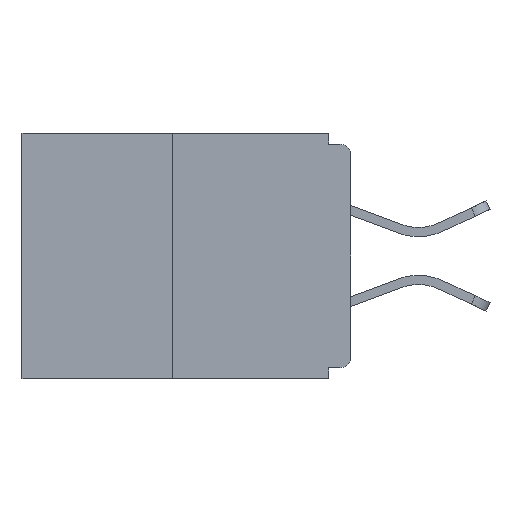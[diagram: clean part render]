
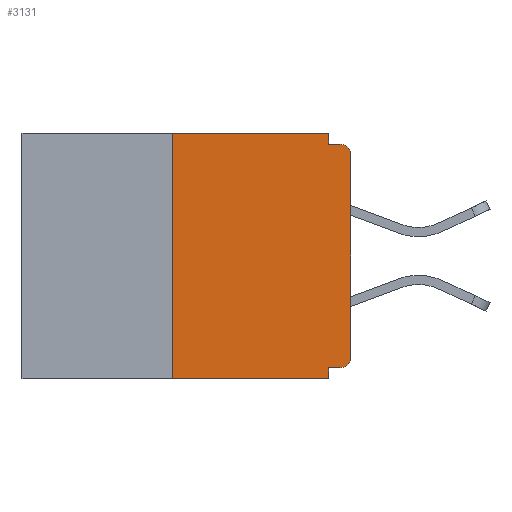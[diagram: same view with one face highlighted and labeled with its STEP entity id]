
A CAD part, left-side view. The second image highlights one B-rep face of the part: STEP entity #3131.
In plain terms, the highlighted planar face has unit normal (-1, 0, 0).
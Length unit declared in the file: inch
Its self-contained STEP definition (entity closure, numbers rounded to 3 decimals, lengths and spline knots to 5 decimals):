
#5 = DIRECTION ( 'NONE',  ( 0., 0., -1. ) ) ;
#140 = CARTESIAN_POINT ( 'NONE',  ( 0., 0.015, -0.03 ) ) ;
#191 = DIRECTION ( 'NONE',  ( 0., 0., -1. ) ) ;
#208 = CARTESIAN_POINT ( 'NONE',  ( 0., 0., -0.313 ) ) ;
#235 = VECTOR ( 'NONE', #4540, 39.37008 ) ;
#478 = EDGE_CURVE ( 'NONE', #4354, #5732, #7126, .T. ) ;
#539 = DIRECTION ( 'NONE',  ( 0., -1., 0. ) ) ;
#550 = EDGE_CURVE ( 'NONE', #5546, #5418, #6744, .T. ) ;
#612 = LINE ( 'NONE', #3067, #3023 ) ;
#686 = ORIENTED_EDGE ( 'NONE', *, *, #10364, .T. ) ;
#1331 = CARTESIAN_POINT ( 'NONE',  ( 0., 0.25, 0. ) ) ;
#1638 = VECTOR ( 'NONE', #6663, 39.37008 ) ;
#1967 = VERTEX_POINT ( 'NONE', #8378 ) ;
#2022 = CIRCLE ( 'NONE', #10120, 0.015 ) ;
#2124 = LINE ( 'NONE', #14376, #12943 ) ;
#2275 = ORIENTED_EDGE ( 'NONE', *, *, #2894, .T. ) ;
#2577 = DIRECTION ( 'NONE',  ( 1., 0., 0. ) ) ;
#2894 = EDGE_CURVE ( 'NONE', #5546, #4735, #2022, .T. ) ;
#2898 = CARTESIAN_POINT ( 'NONE',  ( 0., 0.015, -0.015 ) ) ;
#3023 = VECTOR ( 'NONE', #10588, 39.37008 ) ;
#3067 = CARTESIAN_POINT ( 'NONE',  ( 0., 0.25, 0. ) ) ;
#3131 = ADVANCED_FACE ( 'NONE', ( #10242 ), #11350, .F. ) ;
#3276 = VERTEX_POINT ( 'NONE', #9577 ) ;
#3657 = CARTESIAN_POINT ( 'NONE',  ( 0., 0., -0.015 ) ) ;
#3963 = DIRECTION ( 'NONE',  ( -1., 0., 0. ) ) ;
#4160 = VERTEX_POINT ( 'NONE', #7497 ) ;
#4187 = CARTESIAN_POINT ( 'NONE',  ( 0., 0.015, -0.313 ) ) ;
#4350 = VECTOR ( 'NONE', #9891, 39.37008 ) ;
#4354 = VERTEX_POINT ( 'NONE', #1331 ) ;
#4540 = DIRECTION ( 'NONE',  ( 0., 0., 1. ) ) ;
#4735 = VERTEX_POINT ( 'NONE', #208 ) ;
#5418 = VERTEX_POINT ( 'NONE', #10312 ) ;
#5546 = VERTEX_POINT ( 'NONE', #13089 ) ;
#5732 = VERTEX_POINT ( 'NONE', #11328 ) ;
#5743 = DIRECTION ( 'NONE',  ( 0., 0., -1. ) ) ;
#5886 = CARTESIAN_POINT ( 'NONE',  ( 0., 0.031, 0. ) ) ;
#5913 = ORIENTED_EDGE ( 'NONE', *, *, #6759, .F. ) ;
#5935 = ORIENTED_EDGE ( 'NONE', *, *, #11671, .T. ) ;
#6023 = ORIENTED_EDGE ( 'NONE', *, *, #550, .F. ) ;
#6123 = VECTOR ( 'NONE', #539, 39.37008 ) ;
#6312 = CARTESIAN_POINT ( 'NONE',  ( 0., 0.46, 0. ) ) ;
#6349 = ORIENTED_EDGE ( 'NONE', *, *, #6491, .F. ) ;
#6491 = EDGE_CURVE ( 'NONE', #5418, #1967, #7750, .T. ) ;
#6597 = CARTESIAN_POINT ( 'NONE',  ( 0., 0., -0.328 ) ) ;
#6663 = DIRECTION ( 'NONE',  ( 0., 0., -1. ) ) ;
#6671 = VECTOR ( 'NONE', #5743, 39.37008 ) ;
#6744 = LINE ( 'NONE', #6597, #4350 ) ;
#6759 = EDGE_CURVE ( 'NONE', #7288, #4354, #612, .T. ) ;
#6801 = EDGE_LOOP ( 'NONE', ( #8168, #5913, #686, #6349, #6023, #2275, #5935, #8076, #10536, #8285 ) ) ;
#7126 = LINE ( 'NONE', #6312, #10407 ) ;
#7288 = VERTEX_POINT ( 'NONE', #9785 ) ;
#7497 = CARTESIAN_POINT ( 'NONE',  ( 0., 0., -0.03 ) ) ;
#7750 = LINE ( 'NONE', #7894, #1638 ) ;
#7894 = CARTESIAN_POINT ( 'NONE',  ( 0., 0.031, -0.343 ) ) ;
#8076 = ORIENTED_EDGE ( 'NONE', *, *, #10401, .T. ) ;
#8155 = DIRECTION ( 'NONE',  ( 0., -1., 0. ) ) ;
#8168 = ORIENTED_EDGE ( 'NONE', *, *, #478, .F. ) ;
#8184 = EDGE_CURVE ( 'NONE', #3276, #13270, #10516, .T. ) ;
#8285 = ORIENTED_EDGE ( 'NONE', *, *, #14337, .F. ) ;
#8350 = LINE ( 'NONE', #5886, #6671 ) ;
#8378 = CARTESIAN_POINT ( 'NONE',  ( 0., 0.031, -0.343 ) ) ;
#8497 = AXIS2_PLACEMENT_3D ( 'NONE', #140, #13277, #5 ) ;
#8645 = DIRECTION ( 'NONE',  ( 0., 0., -1. ) ) ;
#9577 = CARTESIAN_POINT ( 'NONE',  ( 0., 0.031, -0.015 ) ) ;
#9785 = CARTESIAN_POINT ( 'NONE',  ( 0., 0.25, -0.343 ) ) ;
#9891 = DIRECTION ( 'NONE',  ( 0., 1., 0. ) ) ;
#10120 = AXIS2_PLACEMENT_3D ( 'NONE', #4187, #3963, #8645 ) ;
#10141 = CIRCLE ( 'NONE', #8497, 0.015 ) ;
#10242 = FACE_OUTER_BOUND ( 'NONE', #6801, .T. ) ;
#10312 = CARTESIAN_POINT ( 'NONE',  ( 0., 0.031, -0.328 ) ) ;
#10319 = CARTESIAN_POINT ( 'NONE',  ( 0., 0., 0. ) ) ;
#10364 = EDGE_CURVE ( 'NONE', #7288, #1967, #2124, .T. ) ;
#10401 = EDGE_CURVE ( 'NONE', #4160, #13270, #10141, .T. ) ;
#10407 = VECTOR ( 'NONE', #8155, 39.37008 ) ;
#10516 = LINE ( 'NONE', #3657, #6123 ) ;
#10536 = ORIENTED_EDGE ( 'NONE', *, *, #8184, .F. ) ;
#10588 = DIRECTION ( 'NONE',  ( 0., 0., 1. ) ) ;
#10951 = DIRECTION ( 'NONE',  ( 0., -1., 0. ) ) ;
#11328 = CARTESIAN_POINT ( 'NONE',  ( 0., 0.031, 0. ) ) ;
#11350 = PLANE ( 'NONE',  #11528 ) ;
#11426 = LINE ( 'NONE', #10319, #235 ) ;
#11528 = AXIS2_PLACEMENT_3D ( 'NONE', #12654, #2577, #191 ) ;
#11671 = EDGE_CURVE ( 'NONE', #4735, #4160, #11426, .T. ) ;
#12654 = CARTESIAN_POINT ( 'NONE',  ( 0., 0.46, 0. ) ) ;
#12943 = VECTOR ( 'NONE', #10951, 39.37008 ) ;
#13089 = CARTESIAN_POINT ( 'NONE',  ( 0., 0.015, -0.328 ) ) ;
#13270 = VERTEX_POINT ( 'NONE', #2898 ) ;
#13277 = DIRECTION ( 'NONE',  ( -1., 0., 0. ) ) ;
#14337 = EDGE_CURVE ( 'NONE', #5732, #3276, #8350, .T. ) ;
#14376 = CARTESIAN_POINT ( 'NONE',  ( 0., 0.46, -0.343 ) ) ;
